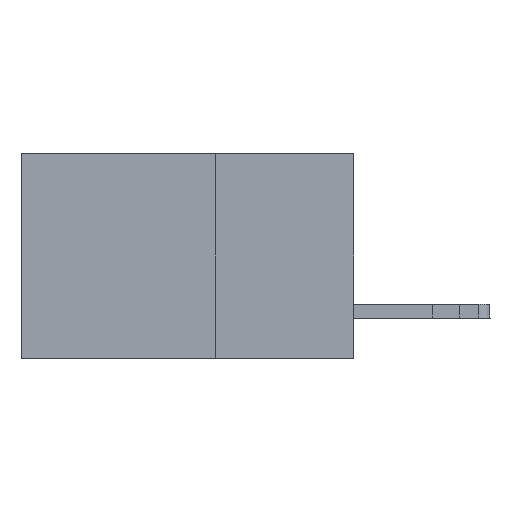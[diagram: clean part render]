
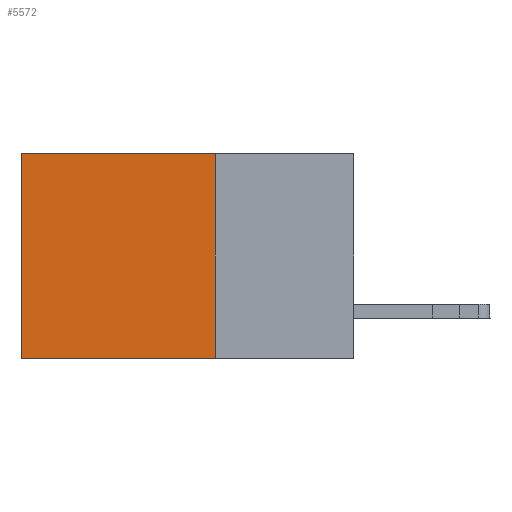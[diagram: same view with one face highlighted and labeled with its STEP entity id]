
A CAD part, left-side view. The second image highlights one B-rep face of the part: STEP entity #5572.
In plain terms, the highlighted planar face has unit normal (-1, 0, 0).
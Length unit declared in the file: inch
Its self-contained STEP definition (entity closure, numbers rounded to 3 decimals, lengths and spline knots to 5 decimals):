
#110 = DIRECTION ( 'NONE',  ( 0., 0., -1. ) ) ;
#164 = VECTOR ( 'NONE', #12758, 39.37008 ) ;
#865 = EDGE_CURVE ( 'NONE', #22028, #15212, #17117, .T. ) ;
#1976 = VECTOR ( 'NONE', #10938, 39.37008 ) ;
#2282 = CARTESIAN_POINT ( 'NONE',  ( 0.2875, 0.25, -0.37 ) ) ;
#2555 = CARTESIAN_POINT ( 'NONE',  ( 0.2875, 0.6, 0. ) ) ;
#2668 = LINE ( 'NONE', #18570, #164 ) ;
#2727 = CARTESIAN_POINT ( 'NONE',  ( 0.2875, 0.25, 0. ) ) ;
#2805 = DIRECTION ( 'NONE',  ( 0., 0., -1. ) ) ;
#2946 = CARTESIAN_POINT ( 'NONE',  ( 0.2875, 0.6, 0. ) ) ;
#4183 = FACE_OUTER_BOUND ( 'NONE', #16397, .T. ) ;
#5572 = ADVANCED_FACE ( 'NONE', ( #4183 ), #24042, .F. ) ;
#6458 = ORIENTED_EDGE ( 'NONE', *, *, #19882, .F. ) ;
#6587 = ORIENTED_EDGE ( 'NONE', *, *, #865, .T. ) ;
#6715 = AXIS2_PLACEMENT_3D ( 'NONE', #12043, #25744, #110 ) ;
#7234 = LINE ( 'NONE', #17460, #8766 ) ;
#7728 = ORIENTED_EDGE ( 'NONE', *, *, #23412, .T. ) ;
#8751 = VERTEX_POINT ( 'NONE', #2282 ) ;
#8766 = VECTOR ( 'NONE', #25257, 39.37008 ) ;
#8993 = EDGE_CURVE ( 'NONE', #17227, #8751, #2668, .T. ) ;
#10938 = DIRECTION ( 'NONE',  ( 0., 1., 0. ) ) ;
#11179 = LINE ( 'NONE', #24894, #1976 ) ;
#12043 = CARTESIAN_POINT ( 'NONE',  ( 0.2875, 0.25, 0. ) ) ;
#12758 = DIRECTION ( 'NONE',  ( 0., 0., -1. ) ) ;
#15212 = VERTEX_POINT ( 'NONE', #15601 ) ;
#15601 = CARTESIAN_POINT ( 'NONE',  ( 0.2875, 0.6, -0.37 ) ) ;
#16397 = EDGE_LOOP ( 'NONE', ( #6587, #6458, #18814, #7728 ) ) ;
#17117 = LINE ( 'NONE', #2946, #25236 ) ;
#17227 = VERTEX_POINT ( 'NONE', #2727 ) ;
#17460 = CARTESIAN_POINT ( 'NONE',  ( 0.2875, 0.25, -0.37 ) ) ;
#18570 = CARTESIAN_POINT ( 'NONE',  ( 0.2875, 0.25, 0. ) ) ;
#18814 = ORIENTED_EDGE ( 'NONE', *, *, #8993, .F. ) ;
#19882 = EDGE_CURVE ( 'NONE', #8751, #15212, #7234, .T. ) ;
#22028 = VERTEX_POINT ( 'NONE', #2555 ) ;
#23412 = EDGE_CURVE ( 'NONE', #17227, #22028, #11179, .T. ) ;
#24042 = PLANE ( 'NONE',  #6715 ) ;
#24894 = CARTESIAN_POINT ( 'NONE',  ( 0.2875, 0.25, 0. ) ) ;
#25236 = VECTOR ( 'NONE', #2805, 39.37008 ) ;
#25257 = DIRECTION ( 'NONE',  ( 0., 1., 0. ) ) ;
#25744 = DIRECTION ( 'NONE',  ( 1., 0., 0. ) ) ;
